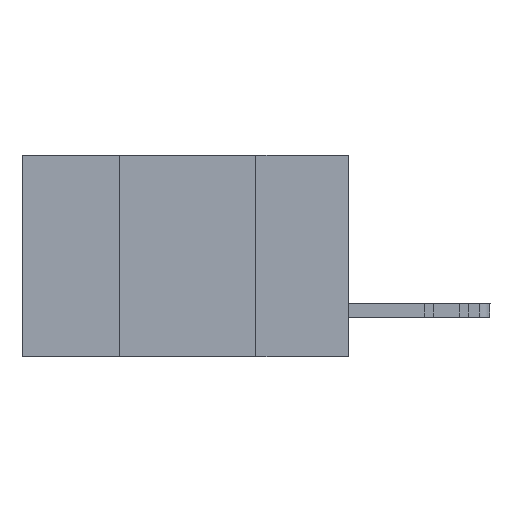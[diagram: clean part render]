
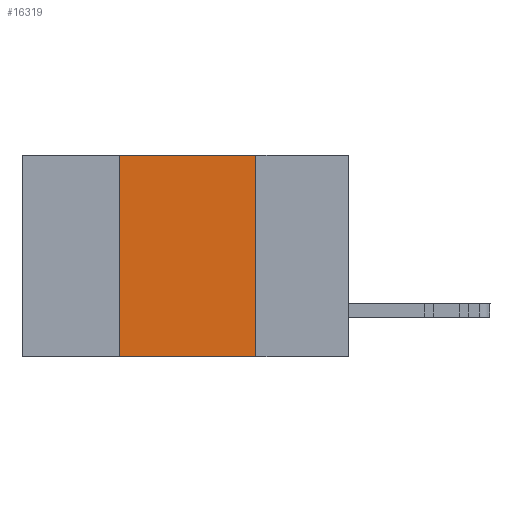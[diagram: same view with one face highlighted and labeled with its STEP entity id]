
A CAD part, left-side view. The second image highlights one B-rep face of the part: STEP entity #16319.
In plain terms, the highlighted planar face has unit normal (-1, 0, 0).
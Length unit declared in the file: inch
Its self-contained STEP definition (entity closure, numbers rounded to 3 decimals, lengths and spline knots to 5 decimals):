
#698 = ORIENTED_EDGE ( 'NONE', *, *, #2047, .F. ) ;
#1133 = DIRECTION ( 'NONE',  ( 0., -1., 0. ) ) ;
#1142 = CARTESIAN_POINT ( 'NONE',  ( 0., 0.42, -0.37 ) ) ;
#1312 = VERTEX_POINT ( 'NONE', #18509 ) ;
#1697 = LINE ( 'NONE', #11504, #2600 ) ;
#1980 = DIRECTION ( 'NONE',  ( 0., -1., 0. ) ) ;
#2047 = EDGE_CURVE ( 'NONE', #5294, #20641, #1697, .T. ) ;
#2060 = LINE ( 'NONE', #22049, #17841 ) ;
#2600 = VECTOR ( 'NONE', #11625, 39.37008 ) ;
#2706 = EDGE_CURVE ( 'NONE', #23252, #1312, #2060, .T. ) ;
#2894 = ORIENTED_EDGE ( 'NONE', *, *, #12890, .F. ) ;
#4198 = DIRECTION ( 'NONE',  ( 0., 0., -1. ) ) ;
#4822 = CARTESIAN_POINT ( 'NONE',  ( 0., 0.17, -0.37 ) ) ;
#5294 = VERTEX_POINT ( 'NONE', #19519 ) ;
#5614 = CARTESIAN_POINT ( 'NONE',  ( 0., 0.6, -0.37 ) ) ;
#6123 = CARTESIAN_POINT ( 'NONE',  ( 0., 0.6, 0. ) ) ;
#8041 = EDGE_CURVE ( 'NONE', #23252, #20641, #11654, .T. ) ;
#9123 = AXIS2_PLACEMENT_3D ( 'NONE', #6123, #13982, #4198 ) ;
#11504 = CARTESIAN_POINT ( 'NONE',  ( 0., 0.17, -0.37 ) ) ;
#11625 = DIRECTION ( 'NONE',  ( 0., 0., -1. ) ) ;
#11654 = LINE ( 'NONE', #5614, #13422 ) ;
#12745 = LINE ( 'NONE', #25000, #17250 ) ;
#12890 = EDGE_CURVE ( 'NONE', #1312, #5294, #12745, .T. ) ;
#13422 = VECTOR ( 'NONE', #1980, 39.37008 ) ;
#13726 = FACE_OUTER_BOUND ( 'NONE', #18780, .T. ) ;
#13982 = DIRECTION ( 'NONE',  ( 1., 0., 0. ) ) ;
#15593 = ORIENTED_EDGE ( 'NONE', *, *, #8041, .T. ) ;
#16319 = ADVANCED_FACE ( 'NONE', ( #13726 ), #19778, .F. ) ;
#16418 = ORIENTED_EDGE ( 'NONE', *, *, #2706, .F. ) ;
#17250 = VECTOR ( 'NONE', #1133, 39.37008 ) ;
#17841 = VECTOR ( 'NONE', #24119, 39.37008 ) ;
#18509 = CARTESIAN_POINT ( 'NONE',  ( 0., 0.42, 0. ) ) ;
#18780 = EDGE_LOOP ( 'NONE', ( #698, #2894, #16418, #15593 ) ) ;
#19519 = CARTESIAN_POINT ( 'NONE',  ( 0., 0.17, 0. ) ) ;
#19778 = PLANE ( 'NONE',  #9123 ) ;
#20641 = VERTEX_POINT ( 'NONE', #4822 ) ;
#22049 = CARTESIAN_POINT ( 'NONE',  ( 0., 0.42, -0.37 ) ) ;
#23252 = VERTEX_POINT ( 'NONE', #1142 ) ;
#24119 = DIRECTION ( 'NONE',  ( 0., 0., 1. ) ) ;
#25000 = CARTESIAN_POINT ( 'NONE',  ( 0., 0.6, 0. ) ) ;
